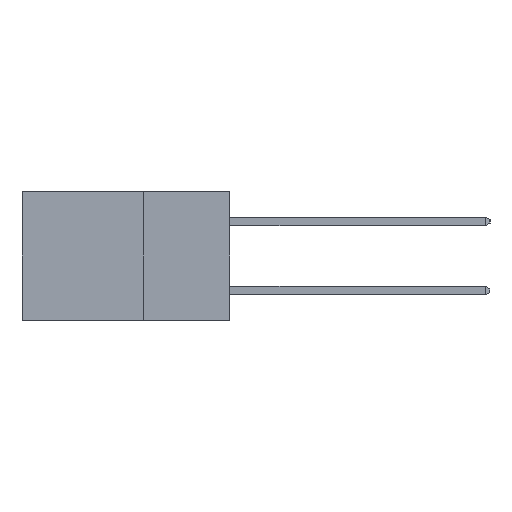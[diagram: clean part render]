
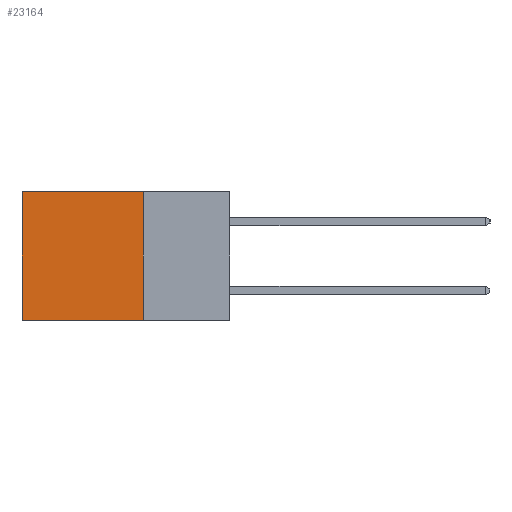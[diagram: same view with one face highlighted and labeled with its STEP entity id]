
A CAD part, left-side view. The second image highlights one B-rep face of the part: STEP entity #23164.
In plain terms, the highlighted planar face has unit normal (-1, 0, 0).
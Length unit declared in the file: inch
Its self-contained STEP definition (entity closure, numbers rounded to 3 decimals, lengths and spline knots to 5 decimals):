
#2273 = ORIENTED_EDGE ( 'NONE', *, *, #9366, .T. ) ;
#3147 = ORIENTED_EDGE ( 'NONE', *, *, #6121, .T. ) ;
#3985 = VECTOR ( 'NONE', #5494, 39.37008 ) ;
#5281 = FACE_OUTER_BOUND ( 'NONE', #13366, .T. ) ;
#5494 = DIRECTION ( 'NONE',  ( 0., 0., -1. ) ) ;
#6121 = EDGE_CURVE ( 'NONE', #23626, #15768, #19981, .T. ) ;
#6470 = ORIENTED_EDGE ( 'NONE', *, *, #16484, .F. ) ;
#7098 = VECTOR ( 'NONE', #21699, 39.37008 ) ;
#9232 = DIRECTION ( 'NONE',  ( 0., 1., 0. ) ) ;
#9366 = EDGE_CURVE ( 'NONE', #9439, #23626, #17072, .T. ) ;
#9439 = VERTEX_POINT ( 'NONE', #22352 ) ;
#10231 = CARTESIAN_POINT ( 'NONE',  ( 0.298, 0.25, 0. ) ) ;
#10385 = CARTESIAN_POINT ( 'NONE',  ( 0.298, 0.6, -0.37 ) ) ;
#10492 = LINE ( 'NONE', #18385, #26305 ) ;
#11361 = VECTOR ( 'NONE', #9232, 39.37008 ) ;
#11866 = DIRECTION ( 'NONE',  ( 0., 1., 0. ) ) ;
#11900 = CARTESIAN_POINT ( 'NONE',  ( 0.298, 0.25, -0.37 ) ) ;
#12361 = DIRECTION ( 'NONE',  ( 0., 0., -1. ) ) ;
#13366 = EDGE_LOOP ( 'NONE', ( #3147, #16362, #6470, #2273 ) ) ;
#14820 = LINE ( 'NONE', #18495, #3985 ) ;
#15768 = VERTEX_POINT ( 'NONE', #10385 ) ;
#15922 = CARTESIAN_POINT ( 'NONE',  ( 0.298, 0.6, 0. ) ) ;
#16362 = ORIENTED_EDGE ( 'NONE', *, *, #22337, .F. ) ;
#16484 = EDGE_CURVE ( 'NONE', #9439, #21621, #14820, .T. ) ;
#17072 = LINE ( 'NONE', #19990, #11361 ) ;
#18385 = CARTESIAN_POINT ( 'NONE',  ( 0.298, 0.25, -0.37 ) ) ;
#18495 = CARTESIAN_POINT ( 'NONE',  ( 0.298, 0.25, 0. ) ) ;
#19981 = LINE ( 'NONE', #20909, #7098 ) ;
#19990 = CARTESIAN_POINT ( 'NONE',  ( 0.298, 0.25, 0. ) ) ;
#20388 = AXIS2_PLACEMENT_3D ( 'NONE', #10231, #25282, #12361 ) ;
#20909 = CARTESIAN_POINT ( 'NONE',  ( 0.298, 0.6, 0. ) ) ;
#21621 = VERTEX_POINT ( 'NONE', #11900 ) ;
#21699 = DIRECTION ( 'NONE',  ( 0., 0., -1. ) ) ;
#22337 = EDGE_CURVE ( 'NONE', #21621, #15768, #10492, .T. ) ;
#22352 = CARTESIAN_POINT ( 'NONE',  ( 0.298, 0.25, 0. ) ) ;
#23164 = ADVANCED_FACE ( 'NONE', ( #5281 ), #25202, .F. ) ;
#23626 = VERTEX_POINT ( 'NONE', #15922 ) ;
#25202 = PLANE ( 'NONE',  #20388 ) ;
#25282 = DIRECTION ( 'NONE',  ( 1., 0., 0. ) ) ;
#26305 = VECTOR ( 'NONE', #11866, 39.37008 ) ;
